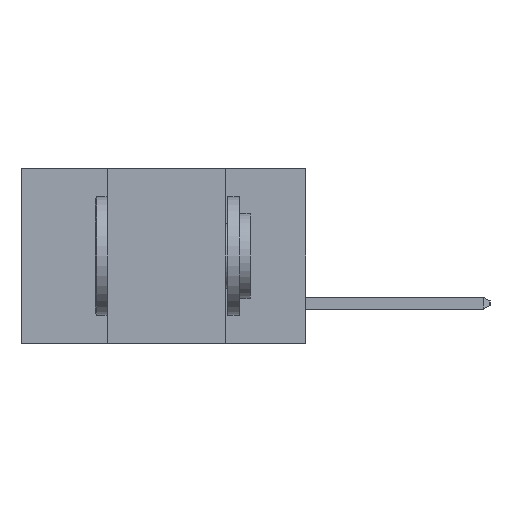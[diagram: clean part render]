
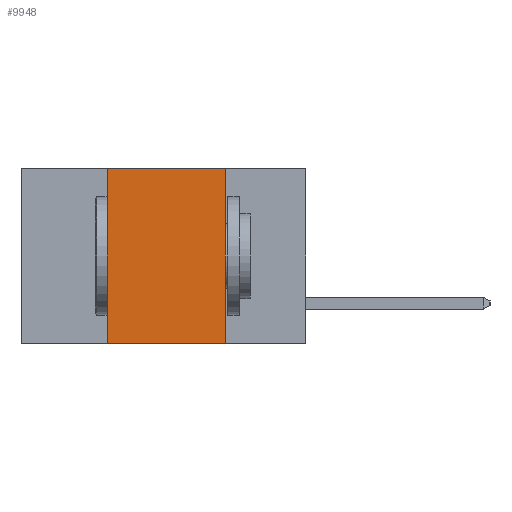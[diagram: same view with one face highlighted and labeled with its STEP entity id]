
A CAD part, left-side view. The second image highlights one B-rep face of the part: STEP entity #9948.
In plain terms, the highlighted planar face has unit normal (-1, 0, 0).
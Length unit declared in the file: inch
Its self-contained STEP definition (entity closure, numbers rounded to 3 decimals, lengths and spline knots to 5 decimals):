
#703 = CARTESIAN_POINT ( 'NONE',  ( 0., 0.42, 0. ) ) ;
#2757 = DIRECTION ( 'NONE',  ( 0., 0., -1. ) ) ;
#2795 = LINE ( 'NONE', #25951, #13511 ) ;
#4551 = VECTOR ( 'NONE', #2757, 39.37008 ) ;
#4869 = VERTEX_POINT ( 'NONE', #24510 ) ;
#4909 = DIRECTION ( 'NONE',  ( 0., -1., 0. ) ) ;
#5435 = EDGE_CURVE ( 'NONE', #15115, #11785, #22024, .T. ) ;
#6247 = CARTESIAN_POINT ( 'NONE',  ( 0., 0.6, -0.37 ) ) ;
#8923 = CARTESIAN_POINT ( 'NONE',  ( 0., 0.42, 0. ) ) ;
#9911 = LINE ( 'NONE', #8923, #22194 ) ;
#9948 = ADVANCED_FACE ( 'NONE', ( #24411 ), #18367, .F. ) ;
#10355 = CARTESIAN_POINT ( 'NONE',  ( 0., 0.17, -0.37 ) ) ;
#11785 = VERTEX_POINT ( 'NONE', #10355 ) ;
#12977 = DIRECTION ( 'NONE',  ( 0., -1., 0. ) ) ;
#13511 = VECTOR ( 'NONE', #12977, 39.37008 ) ;
#14036 = AXIS2_PLACEMENT_3D ( 'NONE', #18334, #18068, #17922 ) ;
#14548 = ORIENTED_EDGE ( 'NONE', *, *, #16369, .F. ) ;
#14880 = VECTOR ( 'NONE', #4909, 39.37008 ) ;
#15115 = VERTEX_POINT ( 'NONE', #17233 ) ;
#16369 = EDGE_CURVE ( 'NONE', #26316, #4869, #2795, .T. ) ;
#17233 = CARTESIAN_POINT ( 'NONE',  ( 0., 0.42, -0.37 ) ) ;
#17922 = DIRECTION ( 'NONE',  ( 0., 0., -1. ) ) ;
#18068 = DIRECTION ( 'NONE',  ( 1., 0., 0. ) ) ;
#18244 = ORIENTED_EDGE ( 'NONE', *, *, #5435, .T. ) ;
#18334 = CARTESIAN_POINT ( 'NONE',  ( 0., 0.6, 0. ) ) ;
#18367 = PLANE ( 'NONE',  #14036 ) ;
#19838 = CARTESIAN_POINT ( 'NONE',  ( 0., 0.17, 0. ) ) ;
#20434 = EDGE_CURVE ( 'NONE', #4869, #11785, #23132, .T. ) ;
#21992 = ORIENTED_EDGE ( 'NONE', *, *, #24844, .F. ) ;
#22023 = ORIENTED_EDGE ( 'NONE', *, *, #20434, .F. ) ;
#22024 = LINE ( 'NONE', #6247, #14880 ) ;
#22194 = VECTOR ( 'NONE', #24144, 39.37008 ) ;
#23132 = LINE ( 'NONE', #19838, #4551 ) ;
#23152 = EDGE_LOOP ( 'NONE', ( #22023, #14548, #21992, #18244 ) ) ;
#24144 = DIRECTION ( 'NONE',  ( 0., 0., 1. ) ) ;
#24411 = FACE_OUTER_BOUND ( 'NONE', #23152, .T. ) ;
#24510 = CARTESIAN_POINT ( 'NONE',  ( 0., 0.17, 0. ) ) ;
#24844 = EDGE_CURVE ( 'NONE', #15115, #26316, #9911, .T. ) ;
#25951 = CARTESIAN_POINT ( 'NONE',  ( 0., 0.6, 0. ) ) ;
#26316 = VERTEX_POINT ( 'NONE', #703 ) ;
